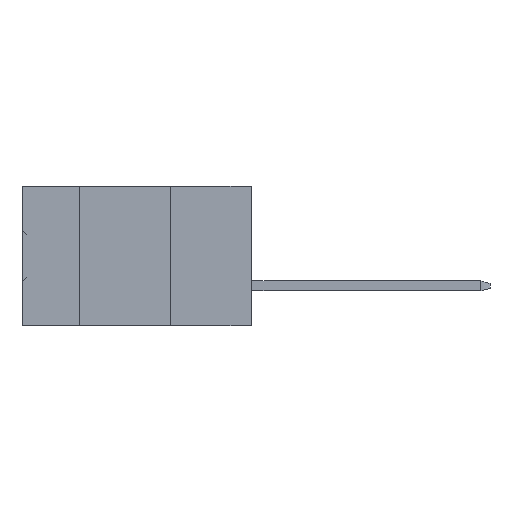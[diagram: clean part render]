
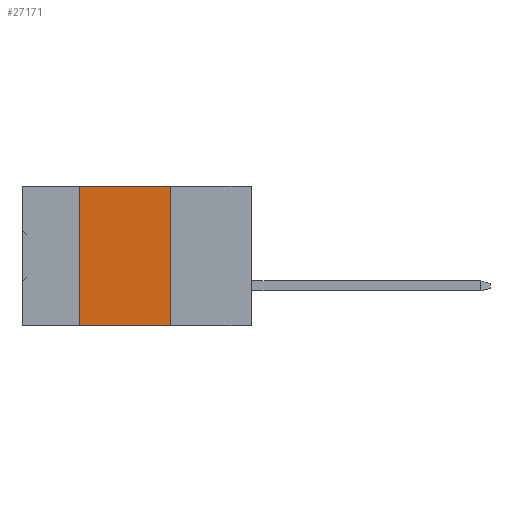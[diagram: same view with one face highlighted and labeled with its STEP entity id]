
A CAD part, left-side view. The second image highlights one B-rep face of the part: STEP entity #27171.
In plain terms, the highlighted planar face has unit normal (-1, 0, 0).
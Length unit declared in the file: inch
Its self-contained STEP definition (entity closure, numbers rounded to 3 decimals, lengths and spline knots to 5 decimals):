
#1073 = EDGE_CURVE ( 'NONE', #23210, #28975, #29349, .T. ) ;
#1094 = ORIENTED_EDGE ( 'NONE', *, *, #13636, .T. ) ;
#2887 = VECTOR ( 'NONE', #21652, 39.37008 ) ;
#3446 = LINE ( 'NONE', #15069, #28574 ) ;
#3852 = CARTESIAN_POINT ( 'NONE',  ( 0., 0.54, 0. ) ) ;
#5754 = VECTOR ( 'NONE', #19337, 39.37008 ) ;
#6646 = VERTEX_POINT ( 'NONE', #11423 ) ;
#6852 = AXIS2_PLACEMENT_3D ( 'NONE', #24376, #9306, #23899 ) ;
#7402 = DIRECTION ( 'NONE',  ( 0., 0., 1. ) ) ;
#8626 = ORIENTED_EDGE ( 'NONE', *, *, #13527, .F. ) ;
#9306 = DIRECTION ( 'NONE',  ( 1., 0., 0. ) ) ;
#11423 = CARTESIAN_POINT ( 'NONE',  ( 0., 0.54, -0.437 ) ) ;
#11869 = CARTESIAN_POINT ( 'NONE',  ( 0., 0.254, -0.437 ) ) ;
#13527 = EDGE_CURVE ( 'NONE', #6646, #28534, #3446, .T. ) ;
#13636 = EDGE_CURVE ( 'NONE', #6646, #28975, #30595, .T. ) ;
#14108 = FACE_OUTER_BOUND ( 'NONE', #17324, .T. ) ;
#15069 = CARTESIAN_POINT ( 'NONE',  ( 0., 0.54, -0.437 ) ) ;
#15522 = ORIENTED_EDGE ( 'NONE', *, *, #23797, .F. ) ;
#17324 = EDGE_LOOP ( 'NONE', ( #20598, #15522, #8626, #1094 ) ) ;
#17392 = LINE ( 'NONE', #29418, #5754 ) ;
#18099 = CARTESIAN_POINT ( 'NONE',  ( 0., 0.72, -0.437 ) ) ;
#19337 = DIRECTION ( 'NONE',  ( 0., -1., 0. ) ) ;
#20598 = ORIENTED_EDGE ( 'NONE', *, *, #1073, .F. ) ;
#21611 = CARTESIAN_POINT ( 'NONE',  ( 0., 0.254, 0. ) ) ;
#21652 = DIRECTION ( 'NONE',  ( 0., 0., -1. ) ) ;
#21930 = VECTOR ( 'NONE', #27879, 39.37008 ) ;
#23187 = CARTESIAN_POINT ( 'NONE',  ( 0., 0.254, -0.437 ) ) ;
#23210 = VERTEX_POINT ( 'NONE', #21611 ) ;
#23797 = EDGE_CURVE ( 'NONE', #28534, #23210, #17392, .T. ) ;
#23899 = DIRECTION ( 'NONE',  ( 0., 0., -1. ) ) ;
#24376 = CARTESIAN_POINT ( 'NONE',  ( 0., 0.72, 0. ) ) ;
#26763 = PLANE ( 'NONE',  #6852 ) ;
#27171 = ADVANCED_FACE ( 'NONE', ( #14108 ), #26763, .F. ) ;
#27879 = DIRECTION ( 'NONE',  ( 0., -1., 0. ) ) ;
#28534 = VERTEX_POINT ( 'NONE', #3852 ) ;
#28574 = VECTOR ( 'NONE', #7402, 39.37008 ) ;
#28975 = VERTEX_POINT ( 'NONE', #23187 ) ;
#29349 = LINE ( 'NONE', #11869, #2887 ) ;
#29418 = CARTESIAN_POINT ( 'NONE',  ( 0., 0.72, 0. ) ) ;
#30595 = LINE ( 'NONE', #18099, #21930 ) ;
